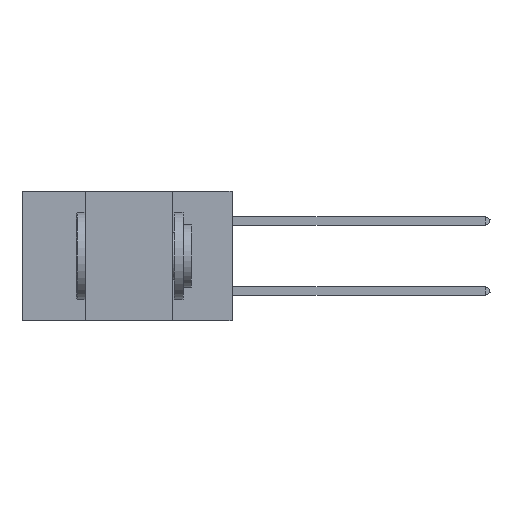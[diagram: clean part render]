
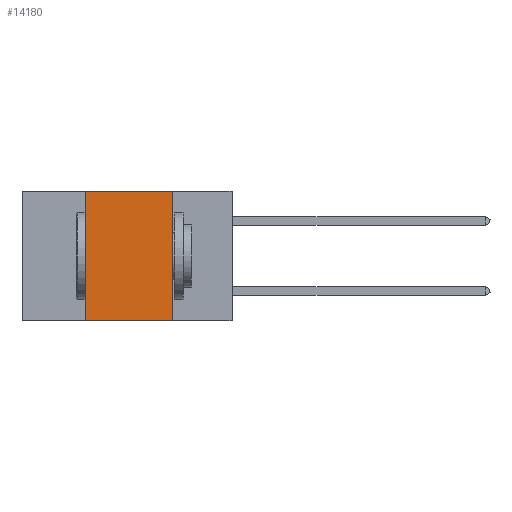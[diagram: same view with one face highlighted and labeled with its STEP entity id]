
A CAD part, left-side view. The second image highlights one B-rep face of the part: STEP entity #14180.
In plain terms, the highlighted planar face has unit normal (-1, 0, 0).
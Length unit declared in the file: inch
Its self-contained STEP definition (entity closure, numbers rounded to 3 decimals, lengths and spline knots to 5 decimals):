
#18 = CARTESIAN_POINT ( 'NONE',  ( 0., 0.6, 0. ) ) ;
#113 = DIRECTION ( 'NONE',  ( 0., -1., 0. ) ) ;
#280 = CARTESIAN_POINT ( 'NONE',  ( 0., 0.17, 0. ) ) ;
#1438 = DIRECTION ( 'NONE',  ( 0., -1., 0. ) ) ;
#2486 = DIRECTION ( 'NONE',  ( 0., 0., -1. ) ) ;
#3118 = VECTOR ( 'NONE', #113, 39.37008 ) ;
#3468 = EDGE_CURVE ( 'NONE', #15707, #9792, #19944, .T. ) ;
#4523 = VERTEX_POINT ( 'NONE', #14438 ) ;
#5645 = LINE ( 'NONE', #14293, #16287 ) ;
#5977 = ORIENTED_EDGE ( 'NONE', *, *, #3468, .F. ) ;
#6257 = EDGE_CURVE ( 'NONE', #9792, #4523, #16915, .T. ) ;
#6698 = FACE_OUTER_BOUND ( 'NONE', #19488, .T. ) ;
#8190 = CARTESIAN_POINT ( 'NONE',  ( 0., 0.42, -0.37 ) ) ;
#9663 = ORIENTED_EDGE ( 'NONE', *, *, #6257, .F. ) ;
#9792 = VERTEX_POINT ( 'NONE', #12016 ) ;
#11284 = DIRECTION ( 'NONE',  ( 1., 0., 0. ) ) ;
#11349 = VECTOR ( 'NONE', #2486, 39.37008 ) ;
#12016 = CARTESIAN_POINT ( 'NONE',  ( 0., 0.17, 0. ) ) ;
#13273 = VECTOR ( 'NONE', #27022, 39.37008 ) ;
#14180 = ADVANCED_FACE ( 'NONE', ( #6698 ), #23720, .F. ) ;
#14293 = CARTESIAN_POINT ( 'NONE',  ( 0., 0.6, -0.37 ) ) ;
#14438 = CARTESIAN_POINT ( 'NONE',  ( 0., 0.17, -0.37 ) ) ;
#15370 = EDGE_CURVE ( 'NONE', #18709, #4523, #5645, .T. ) ;
#15707 = VERTEX_POINT ( 'NONE', #25635 ) ;
#16287 = VECTOR ( 'NONE', #1438, 39.37008 ) ;
#16915 = LINE ( 'NONE', #280, #11349 ) ;
#17900 = ORIENTED_EDGE ( 'NONE', *, *, #20864, .F. ) ;
#18709 = VERTEX_POINT ( 'NONE', #8190 ) ;
#18745 = LINE ( 'NONE', #20795, #13273 ) ;
#19488 = EDGE_LOOP ( 'NONE', ( #9663, #5977, #17900, #24033 ) ) ;
#19944 = LINE ( 'NONE', #18, #3118 ) ;
#20795 = CARTESIAN_POINT ( 'NONE',  ( 0., 0.42, 0. ) ) ;
#20864 = EDGE_CURVE ( 'NONE', #18709, #15707, #18745, .T. ) ;
#22100 = AXIS2_PLACEMENT_3D ( 'NONE', #25691, #11284, #25782 ) ;
#23720 = PLANE ( 'NONE',  #22100 ) ;
#24033 = ORIENTED_EDGE ( 'NONE', *, *, #15370, .T. ) ;
#25635 = CARTESIAN_POINT ( 'NONE',  ( 0., 0.42, 0. ) ) ;
#25691 = CARTESIAN_POINT ( 'NONE',  ( 0., 0.6, 0. ) ) ;
#25782 = DIRECTION ( 'NONE',  ( 0., 0., -1. ) ) ;
#27022 = DIRECTION ( 'NONE',  ( 0., 0., 1. ) ) ;
